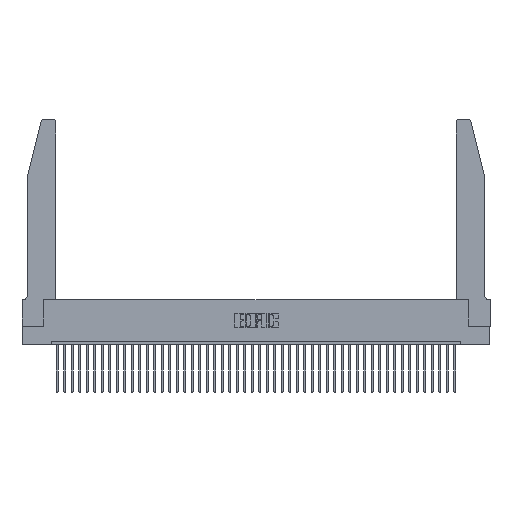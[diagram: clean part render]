
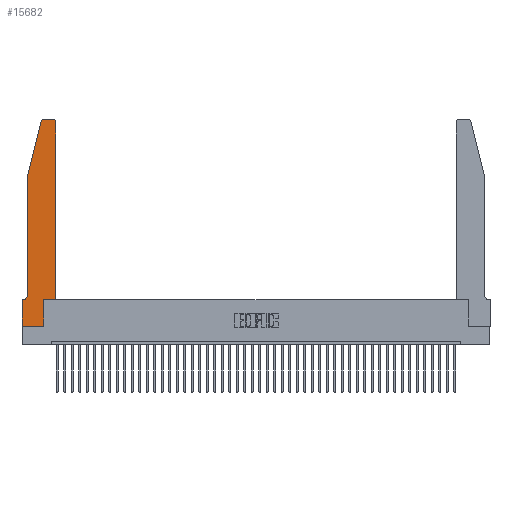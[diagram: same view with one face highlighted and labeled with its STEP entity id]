
A CAD part, top view. The second image highlights one B-rep face of the part: STEP entity #15682.
In plain terms, the highlighted planar face has unit normal (0, 0, 1).
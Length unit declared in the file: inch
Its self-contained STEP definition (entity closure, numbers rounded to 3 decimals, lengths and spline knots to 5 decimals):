
#143 = DIRECTION ( 'NONE',  ( -1., 0., 0. ) ) ;
#184 = CARTESIAN_POINT ( 'NONE',  ( 0.0055, 0.42, 0.37 ) ) ;
#418 = DIRECTION ( 'NONE',  ( 1., 0., 0. ) ) ;
#1571 = CARTESIAN_POINT ( 'NONE',  ( 0.2865, 0., 0.37 ) ) ;
#2027 = LINE ( 'NONE', #37241, #13171 ) ;
#2768 = DIRECTION ( 'NONE',  ( 0., -1., 0. ) ) ;
#2917 = EDGE_CURVE ( 'NONE', #19664, #12896, #12019, .T. ) ;
#3279 = DIRECTION ( 'NONE',  ( -1., 0., 0. ) ) ;
#3740 = PLANE ( 'NONE',  #39458 ) ;
#4165 = CARTESIAN_POINT ( 'NONE',  ( 0., 0., 0.37 ) ) ;
#4509 = LINE ( 'NONE', #30139, #26737 ) ;
#5765 = VECTOR ( 'NONE', #2768, 39.37008 ) ;
#5953 = CARTESIAN_POINT ( 'NONE',  ( 0.284, 2.72, 0.37 ) ) ;
#6168 = CARTESIAN_POINT ( 'NONE',  ( 0., 0.35, 0.37 ) ) ;
#6730 = EDGE_CURVE ( 'NONE', #13266, #25687, #39691, .T. ) ;
#7022 = VERTEX_POINT ( 'NONE', #1571 ) ;
#7058 = DIRECTION ( 'NONE',  ( 0., 0., 1. ) ) ;
#7077 = DIRECTION ( 'NONE',  ( 0., 1., 0. ) ) ;
#7520 = CARTESIAN_POINT ( 'NONE',  ( 0.2865, 0.35, 0.37 ) ) ;
#8390 = EDGE_CURVE ( 'NONE', #12896, #28461, #2027, .T. ) ;
#8541 = ORIENTED_EDGE ( 'NONE', *, *, #8390, .T. ) ;
#10217 = DIRECTION ( 'NONE',  ( 1., 0., 0. ) ) ;
#10463 = ORIENTED_EDGE ( 'NONE', *, *, #12240, .T. ) ;
#10840 = CARTESIAN_POINT ( 'NONE',  ( 0.0755, 2., 0.37 ) ) ;
#11043 = CIRCLE ( 'NONE', #37757, 0.03 ) ;
#11173 = LINE ( 'NONE', #31641, #21725 ) ;
#11480 = ORIENTED_EDGE ( 'NONE', *, *, #6730, .T. ) ;
#12019 = LINE ( 'NONE', #10840, #27338 ) ;
#12240 = EDGE_CURVE ( 'NONE', #28461, #16495, #36308, .T. ) ;
#12466 = LINE ( 'NONE', #7520, #25685 ) ;
#12896 = VERTEX_POINT ( 'NONE', #19804 ) ;
#13171 = VECTOR ( 'NONE', #23848, 39.37008 ) ;
#13266 = VERTEX_POINT ( 'NONE', #18583 ) ;
#13893 = CIRCLE ( 'NONE', #29271, 0.03 ) ;
#14313 = DIRECTION ( 'NONE',  ( -1., 0., 0. ) ) ;
#14741 = CARTESIAN_POINT ( 'NONE',  ( 0.4505, 0.35, 0.37 ) ) ;
#15156 = EDGE_CURVE ( 'NONE', #35670, #13266, #13893, .T. ) ;
#15606 = DIRECTION ( 'NONE',  ( 1., 0., 0. ) ) ;
#15682 = ADVANCED_FACE ( 'NONE', ( #16488 ), #3740, .T. ) ;
#16488 = FACE_OUTER_BOUND ( 'NONE', #30050, .T. ) ;
#16495 = VERTEX_POINT ( 'NONE', #39569 ) ;
#17391 = LINE ( 'NONE', #36439, #5765 ) ;
#17497 = EDGE_CURVE ( 'NONE', #25687, #19664, #11043, .T. ) ;
#17611 = AXIS2_PLACEMENT_3D ( 'NONE', #184, #33568, #3279 ) ;
#17654 = CARTESIAN_POINT ( 'NONE',  ( 0.4505, 2.72, 0.37 ) ) ;
#18583 = CARTESIAN_POINT ( 'NONE',  ( 0.4205, 2.75, 0.37 ) ) ;
#19163 = CARTESIAN_POINT ( 'NONE',  ( 0.0755, 0.42, 0.37 ) ) ;
#19664 = VERTEX_POINT ( 'NONE', #34569 ) ;
#19804 = CARTESIAN_POINT ( 'NONE',  ( 0.0755, 2., 0.37 ) ) ;
#21126 = ORIENTED_EDGE ( 'NONE', *, *, #40756, .T. ) ;
#21725 = VECTOR ( 'NONE', #34438, 39.37008 ) ;
#21810 = VERTEX_POINT ( 'NONE', #34715 ) ;
#22306 = ORIENTED_EDGE ( 'NONE', *, *, #32177, .T. ) ;
#23518 = VECTOR ( 'NONE', #10217, 39.37008 ) ;
#23848 = DIRECTION ( 'NONE',  ( 0., -1., 0. ) ) ;
#25602 = VERTEX_POINT ( 'NONE', #4165 ) ;
#25685 = VECTOR ( 'NONE', #7077, 39.37008 ) ;
#25687 = VERTEX_POINT ( 'NONE', #25744 ) ;
#25744 = CARTESIAN_POINT ( 'NONE',  ( 0.284, 2.75, 0.37 ) ) ;
#25800 = ORIENTED_EDGE ( 'NONE', *, *, #15156, .T. ) ;
#26390 = CARTESIAN_POINT ( 'NONE',  ( 0.4505, 0.35, 0.37 ) ) ;
#26522 = DIRECTION ( 'NONE',  ( 0., 1., 0. ) ) ;
#26737 = VECTOR ( 'NONE', #143, 39.37008 ) ;
#27338 = VECTOR ( 'NONE', #37245, 39.37008 ) ;
#27565 = VECTOR ( 'NONE', #26522, 39.37008 ) ;
#27674 = DIRECTION ( 'NONE',  ( 0., 0., 1. ) ) ;
#27771 = EDGE_CURVE ( 'NONE', #31249, #25602, #17391, .T. ) ;
#28461 = VERTEX_POINT ( 'NONE', #19163 ) ;
#28647 = LINE ( 'NONE', #26390, #27565 ) ;
#29271 = AXIS2_PLACEMENT_3D ( 'NONE', #37894, #7058, #418 ) ;
#30050 = EDGE_LOOP ( 'NONE', ( #11480, #41863, #40188, #8541, #10463, #22306, #30227, #31199, #32910, #21126, #32020, #25800 ) ) ;
#30139 = CARTESIAN_POINT ( 'NONE',  ( 0.0755, 0.35, 0.37 ) ) ;
#30227 = ORIENTED_EDGE ( 'NONE', *, *, #27771, .T. ) ;
#31199 = ORIENTED_EDGE ( 'NONE', *, *, #39049, .T. ) ;
#31249 = VERTEX_POINT ( 'NONE', #6168 ) ;
#31641 = CARTESIAN_POINT ( 'NONE',  ( 0.4505, 0.35, 0.37 ) ) ;
#31811 = DIRECTION ( 'NONE',  ( 1., 0., 0. ) ) ;
#32020 = ORIENTED_EDGE ( 'NONE', *, *, #40430, .T. ) ;
#32177 = EDGE_CURVE ( 'NONE', #16495, #31249, #4509, .T. ) ;
#32294 = EDGE_CURVE ( 'NONE', #7022, #21810, #12466, .T. ) ;
#32692 = DIRECTION ( 'NONE',  ( 0., 0., 1. ) ) ;
#32910 = ORIENTED_EDGE ( 'NONE', *, *, #32294, .T. ) ;
#33568 = DIRECTION ( 'NONE',  ( 0., 0., -1. ) ) ;
#34438 = DIRECTION ( 'NONE',  ( 1., 0., 0. ) ) ;
#34569 = CARTESIAN_POINT ( 'NONE',  ( 0.25487, 2.72718, 0.37 ) ) ;
#34715 = CARTESIAN_POINT ( 'NONE',  ( 0.2865, 0.35, 0.37 ) ) ;
#35670 = VERTEX_POINT ( 'NONE', #17654 ) ;
#36308 = CIRCLE ( 'NONE', #17611, 0.07 ) ;
#36439 = CARTESIAN_POINT ( 'NONE',  ( 0., 0., 0.37 ) ) ;
#37241 = CARTESIAN_POINT ( 'NONE',  ( 0.0755, 2., 0.37 ) ) ;
#37245 = DIRECTION ( 'NONE',  ( -0.239, -0.971, 0. ) ) ;
#37529 = VECTOR ( 'NONE', #14313, 39.37008 ) ;
#37757 = AXIS2_PLACEMENT_3D ( 'NONE', #5953, #32692, #15606 ) ;
#37894 = CARTESIAN_POINT ( 'NONE',  ( 0.4205, 2.72, 0.37 ) ) ;
#38143 = VERTEX_POINT ( 'NONE', #14741 ) ;
#39049 = EDGE_CURVE ( 'NONE', #25602, #7022, #41448, .T. ) ;
#39458 = AXIS2_PLACEMENT_3D ( 'NONE', #40963, #27674, #31811 ) ;
#39569 = CARTESIAN_POINT ( 'NONE',  ( 0.0055, 0.35, 0.37 ) ) ;
#39691 = LINE ( 'NONE', #41174, #37529 ) ;
#40188 = ORIENTED_EDGE ( 'NONE', *, *, #2917, .T. ) ;
#40430 = EDGE_CURVE ( 'NONE', #38143, #35670, #28647, .T. ) ;
#40475 = CARTESIAN_POINT ( 'NONE',  ( 0., 0., 0.37 ) ) ;
#40756 = EDGE_CURVE ( 'NONE', #21810, #38143, #11173, .T. ) ;
#40963 = CARTESIAN_POINT ( 'NONE',  ( 0., 0.35, 0.37 ) ) ;
#41174 = CARTESIAN_POINT ( 'NONE',  ( 0.2605, 2.75, 0.37 ) ) ;
#41448 = LINE ( 'NONE', #40475, #23518 ) ;
#41863 = ORIENTED_EDGE ( 'NONE', *, *, #17497, .T. ) ;
